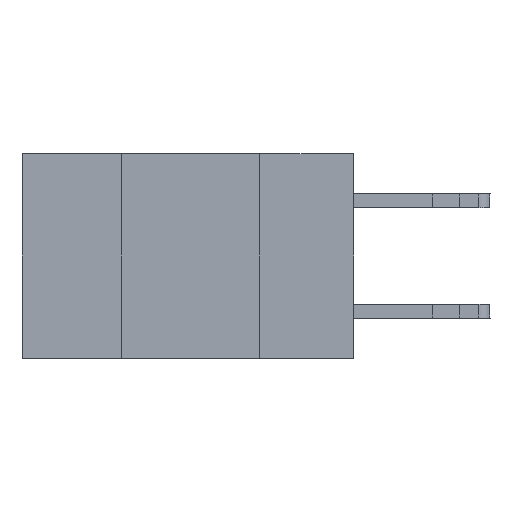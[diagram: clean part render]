
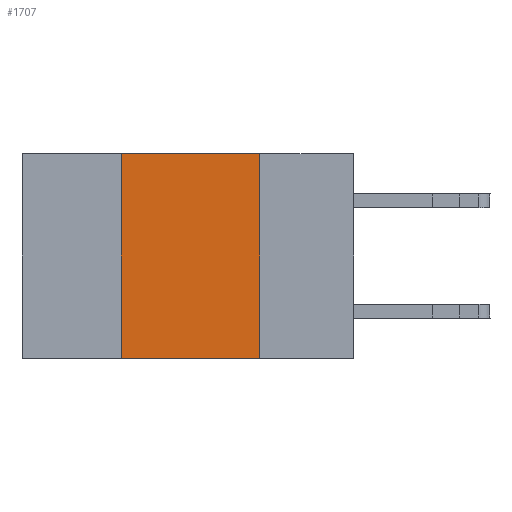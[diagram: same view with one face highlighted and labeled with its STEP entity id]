
A CAD part, left-side view. The second image highlights one B-rep face of the part: STEP entity #1707.
In plain terms, the highlighted planar face has unit normal (-1, 0, 0).
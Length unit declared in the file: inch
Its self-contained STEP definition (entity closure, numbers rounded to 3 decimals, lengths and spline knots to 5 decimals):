
#870 = CARTESIAN_POINT ( 'NONE',  ( 0., 0.6, -0.37 ) ) ;
#949 = VERTEX_POINT ( 'NONE', #6554 ) ;
#1707 = ADVANCED_FACE ( 'NONE', ( #21569 ), #2108, .F. ) ;
#2108 = PLANE ( 'NONE',  #18368 ) ;
#4005 = DIRECTION ( 'NONE',  ( 0., -1., 0. ) ) ;
#5161 = LINE ( 'NONE', #26992, #16918 ) ;
#5702 = EDGE_CURVE ( 'NONE', #14401, #25941, #6318, .T. ) ;
#6318 = LINE ( 'NONE', #16588, #24283 ) ;
#6554 = CARTESIAN_POINT ( 'NONE',  ( 0., 0.17, 0. ) ) ;
#8162 = EDGE_CURVE ( 'NONE', #14401, #8744, #9752, .T. ) ;
#8287 = VECTOR ( 'NONE', #15167, 39.37008 ) ;
#8744 = VERTEX_POINT ( 'NONE', #18250 ) ;
#9752 = LINE ( 'NONE', #870, #8287 ) ;
#10133 = ORIENTED_EDGE ( 'NONE', *, *, #8162, .T. ) ;
#10620 = ORIENTED_EDGE ( 'NONE', *, *, #29701, .F. ) ;
#11733 = DIRECTION ( 'NONE',  ( 0., 0., 1. ) ) ;
#12803 = EDGE_CURVE ( 'NONE', #25941, #949, #5161, .T. ) ;
#13647 = CARTESIAN_POINT ( 'NONE',  ( 0., 0.42, -0.37 ) ) ;
#13978 = EDGE_LOOP ( 'NONE', ( #10620, #25646, #28468, #10133 ) ) ;
#14401 = VERTEX_POINT ( 'NONE', #13647 ) ;
#14740 = CARTESIAN_POINT ( 'NONE',  ( 0., 0.17, 0. ) ) ;
#15167 = DIRECTION ( 'NONE',  ( 0., -1., 0. ) ) ;
#16588 = CARTESIAN_POINT ( 'NONE',  ( 0., 0.42, 0. ) ) ;
#16858 = VECTOR ( 'NONE', #26683, 39.37008 ) ;
#16918 = VECTOR ( 'NONE', #4005, 39.37008 ) ;
#16997 = CARTESIAN_POINT ( 'NONE',  ( 0., 0.42, 0. ) ) ;
#18250 = CARTESIAN_POINT ( 'NONE',  ( 0., 0.17, -0.37 ) ) ;
#18368 = AXIS2_PLACEMENT_3D ( 'NONE', #30368, #30251, #23221 ) ;
#18706 = LINE ( 'NONE', #14740, #16858 ) ;
#21569 = FACE_OUTER_BOUND ( 'NONE', #13978, .T. ) ;
#23221 = DIRECTION ( 'NONE',  ( 0., 0., -1. ) ) ;
#24283 = VECTOR ( 'NONE', #11733, 39.37008 ) ;
#25646 = ORIENTED_EDGE ( 'NONE', *, *, #12803, .F. ) ;
#25941 = VERTEX_POINT ( 'NONE', #16997 ) ;
#26683 = DIRECTION ( 'NONE',  ( 0., 0., -1. ) ) ;
#26992 = CARTESIAN_POINT ( 'NONE',  ( 0., 0.6, 0. ) ) ;
#28468 = ORIENTED_EDGE ( 'NONE', *, *, #5702, .F. ) ;
#29701 = EDGE_CURVE ( 'NONE', #949, #8744, #18706, .T. ) ;
#30251 = DIRECTION ( 'NONE',  ( 1., 0., 0. ) ) ;
#30368 = CARTESIAN_POINT ( 'NONE',  ( 0., 0.6, 0. ) ) ;
